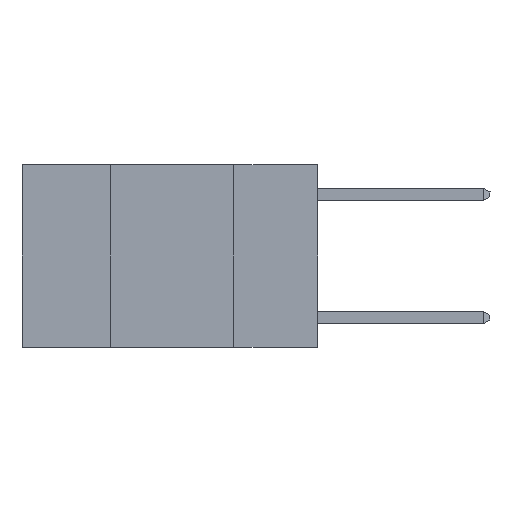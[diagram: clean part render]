
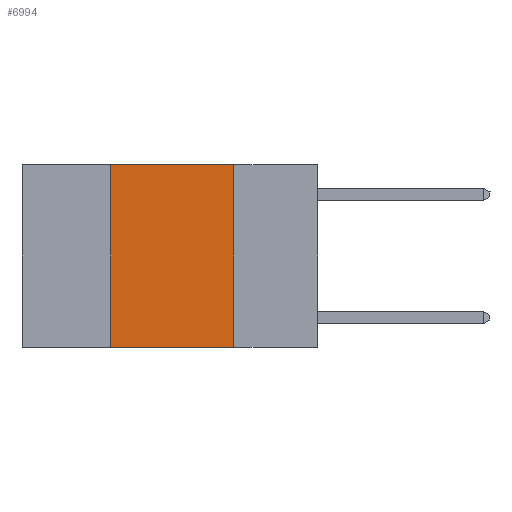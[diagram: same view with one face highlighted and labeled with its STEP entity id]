
A CAD part, left-side view. The second image highlights one B-rep face of the part: STEP entity #6994.
In plain terms, the highlighted planar face has unit normal (-1, 0, 0).
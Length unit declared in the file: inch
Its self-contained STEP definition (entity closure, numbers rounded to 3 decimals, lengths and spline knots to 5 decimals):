
#314 = CARTESIAN_POINT ( 'NONE',  ( 0., 0.17, -0.37 ) ) ;
#386 = FACE_OUTER_BOUND ( 'NONE', #463, .T. ) ;
#463 = EDGE_LOOP ( 'NONE', ( #10580, #1711, #4838, #7883 ) ) ;
#497 = CARTESIAN_POINT ( 'NONE',  ( 0., 0.17, 0. ) ) ;
#1343 = DIRECTION ( 'NONE',  ( 1., 0., 0. ) ) ;
#1711 = ORIENTED_EDGE ( 'NONE', *, *, #8862, .F. ) ;
#2660 = CARTESIAN_POINT ( 'NONE',  ( 0., 0.42, 0. ) ) ;
#2781 = LINE ( 'NONE', #8277, #8568 ) ;
#3233 = CARTESIAN_POINT ( 'NONE',  ( 0., 0.17, 0. ) ) ;
#3304 = LINE ( 'NONE', #497, #12063 ) ;
#3703 = CARTESIAN_POINT ( 'NONE',  ( 0., 0.42, -0.37 ) ) ;
#3889 = CARTESIAN_POINT ( 'NONE',  ( 0., 0.6, -0.37 ) ) ;
#4428 = VECTOR ( 'NONE', #10767, 39.37008 ) ;
#4780 = EDGE_CURVE ( 'NONE', #12794, #11017, #7490, .T. ) ;
#4838 = ORIENTED_EDGE ( 'NONE', *, *, #4843, .F. ) ;
#4843 = EDGE_CURVE ( 'NONE', #12794, #13674, #12420, .T. ) ;
#4868 = EDGE_CURVE ( 'NONE', #13240, #11017, #3304, .T. ) ;
#5175 = CARTESIAN_POINT ( 'NONE',  ( 0., 0.42, 0. ) ) ;
#6994 = ADVANCED_FACE ( 'NONE', ( #386 ), #8322, .F. ) ;
#7490 = LINE ( 'NONE', #3889, #4428 ) ;
#7883 = ORIENTED_EDGE ( 'NONE', *, *, #4780, .T. ) ;
#8277 = CARTESIAN_POINT ( 'NONE',  ( 0., 0.6, 0. ) ) ;
#8322 = PLANE ( 'NONE',  #8768 ) ;
#8568 = VECTOR ( 'NONE', #9449, 39.37008 ) ;
#8659 = DIRECTION ( 'NONE',  ( 0., 0., -1. ) ) ;
#8768 = AXIS2_PLACEMENT_3D ( 'NONE', #13833, #1343, #9489 ) ;
#8862 = EDGE_CURVE ( 'NONE', #13674, #13240, #2781, .T. ) ;
#9449 = DIRECTION ( 'NONE',  ( 0., -1., 0. ) ) ;
#9470 = VECTOR ( 'NONE', #14109, 39.37008 ) ;
#9489 = DIRECTION ( 'NONE',  ( 0., 0., -1. ) ) ;
#10580 = ORIENTED_EDGE ( 'NONE', *, *, #4868, .F. ) ;
#10767 = DIRECTION ( 'NONE',  ( 0., -1., 0. ) ) ;
#11017 = VERTEX_POINT ( 'NONE', #314 ) ;
#12063 = VECTOR ( 'NONE', #8659, 39.37008 ) ;
#12420 = LINE ( 'NONE', #5175, #9470 ) ;
#12794 = VERTEX_POINT ( 'NONE', #3703 ) ;
#13240 = VERTEX_POINT ( 'NONE', #3233 ) ;
#13674 = VERTEX_POINT ( 'NONE', #2660 ) ;
#13833 = CARTESIAN_POINT ( 'NONE',  ( 0., 0.6, 0. ) ) ;
#14109 = DIRECTION ( 'NONE',  ( 0., 0., 1. ) ) ;
